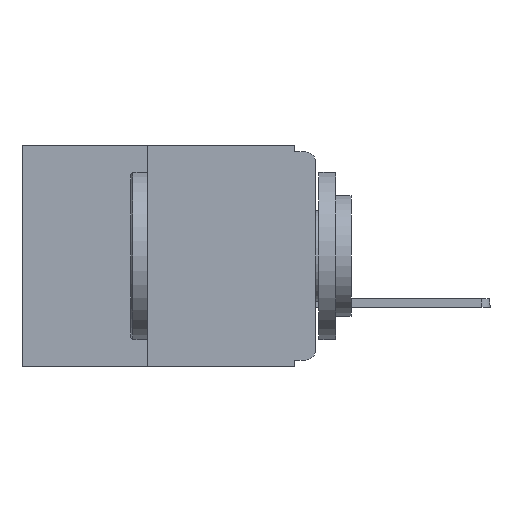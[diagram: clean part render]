
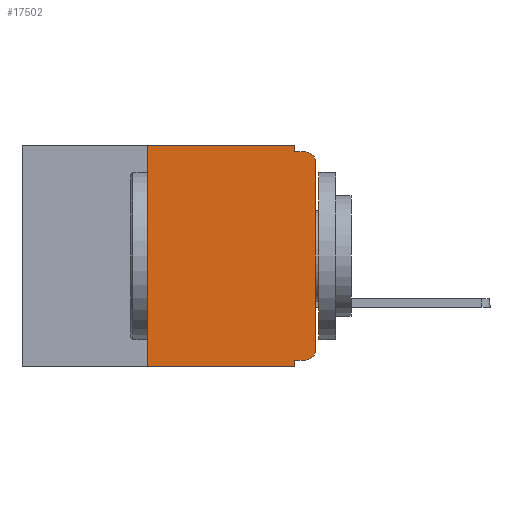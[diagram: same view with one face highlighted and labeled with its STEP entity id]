
A CAD part, left-side view. The second image highlights one B-rep face of the part: STEP entity #17502.
In plain terms, the highlighted planar face has unit normal (-1, 0, 0).
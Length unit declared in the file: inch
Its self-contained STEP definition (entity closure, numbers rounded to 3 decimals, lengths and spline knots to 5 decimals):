
#1093 = ORIENTED_EDGE ( 'NONE', *, *, #18024, .T. ) ;
#1341 = ORIENTED_EDGE ( 'NONE', *, *, #11001, .F. ) ;
#1710 = CARTESIAN_POINT ( 'NONE',  ( 0., 0.015, -0.025 ) ) ;
#1848 = CARTESIAN_POINT ( 'NONE',  ( 0., 0.015, -0.01 ) ) ;
#1984 = VERTEX_POINT ( 'NONE', #11458 ) ;
#2075 = CARTESIAN_POINT ( 'NONE',  ( 0., 0.031, 0. ) ) ;
#2078 = VERTEX_POINT ( 'NONE', #12396 ) ;
#2118 = ORIENTED_EDGE ( 'NONE', *, *, #21403, .F. ) ;
#3249 = ORIENTED_EDGE ( 'NONE', *, *, #15613, .F. ) ;
#3299 = LINE ( 'NONE', #16524, #12833 ) ;
#3483 = AXIS2_PLACEMENT_3D ( 'NONE', #1710, #14924, #3572 ) ;
#3572 = DIRECTION ( 'NONE',  ( 0., 0., -1. ) ) ;
#3679 = VERTEX_POINT ( 'NONE', #23639 ) ;
#3843 = VECTOR ( 'NONE', #21231, 39.37008 ) ;
#4228 = ORIENTED_EDGE ( 'NONE', *, *, #22177, .T. ) ;
#4853 = CARTESIAN_POINT ( 'NONE',  ( 0., 0., 0. ) ) ;
#5460 = DIRECTION ( 'NONE',  ( 0., 0., -1. ) ) ;
#5711 = AXIS2_PLACEMENT_3D ( 'NONE', #20771, #22678, #11487 ) ;
#6062 = CARTESIAN_POINT ( 'NONE',  ( 0., 0., -0.01 ) ) ;
#6402 = EDGE_LOOP ( 'NONE', ( #4228, #1093, #1341, #2118, #3249, #6449, #6737, #7347, #7793, #21954 ) ) ;
#6422 = EDGE_CURVE ( 'NONE', #16972, #3679, #21775, .T. ) ;
#6449 = ORIENTED_EDGE ( 'NONE', *, *, #18558, .F. ) ;
#6737 = ORIENTED_EDGE ( 'NONE', *, *, #16997, .T. ) ;
#7347 = ORIENTED_EDGE ( 'NONE', *, *, #11310, .F. ) ;
#7634 = PLANE ( 'NONE',  #5711 ) ;
#7793 = ORIENTED_EDGE ( 'NONE', *, *, #11449, .F. ) ;
#7931 = VECTOR ( 'NONE', #17489, 39.37008 ) ;
#8108 = CARTESIAN_POINT ( 'NONE',  ( 0., 0.437, 0. ) ) ;
#9319 = VERTEX_POINT ( 'NONE', #21881 ) ;
#9547 = LINE ( 'NONE', #6062, #3843 ) ;
#9656 = DIRECTION ( 'NONE',  ( 0., 1., 0. ) ) ;
#9844 = CARTESIAN_POINT ( 'NONE',  ( 0., 0., -0.025 ) ) ;
#10036 = DIRECTION ( 'NONE',  ( 0., -1., 0. ) ) ;
#10295 = VECTOR ( 'NONE', #18039, 39.37008 ) ;
#10493 = LINE ( 'NONE', #20041, #24250 ) ;
#10742 = DIRECTION ( 'NONE',  ( 0., -1., 0. ) ) ;
#10802 = VERTEX_POINT ( 'NONE', #1848 ) ;
#11001 = EDGE_CURVE ( 'NONE', #1984, #10802, #9547, .T. ) ;
#11310 = EDGE_CURVE ( 'NONE', #2078, #23770, #21860, .T. ) ;
#11338 = CIRCLE ( 'NONE', #3483, 0.015 ) ;
#11449 = EDGE_CURVE ( 'NONE', #16972, #2078, #14525, .T. ) ;
#11458 = CARTESIAN_POINT ( 'NONE',  ( 0., 0.031, -0.01 ) ) ;
#11487 = DIRECTION ( 'NONE',  ( 0., 0., -1. ) ) ;
#11511 = CARTESIAN_POINT ( 'NONE',  ( 0., 0., -0.32 ) ) ;
#11917 = CARTESIAN_POINT ( 'NONE',  ( 0., 0.031, 0. ) ) ;
#12396 = CARTESIAN_POINT ( 'NONE',  ( 0., 0.031, -0.32 ) ) ;
#12606 = LINE ( 'NONE', #8108, #16910 ) ;
#12833 = VECTOR ( 'NONE', #24019, 39.37008 ) ;
#12975 = LINE ( 'NONE', #11917, #7931 ) ;
#13433 = CARTESIAN_POINT ( 'NONE',  ( 0., 0.25, 0. ) ) ;
#13948 = VECTOR ( 'NONE', #9656, 39.37008 ) ;
#14525 = LINE ( 'NONE', #11511, #13948 ) ;
#14906 = VERTEX_POINT ( 'NONE', #13433 ) ;
#14924 = DIRECTION ( 'NONE',  ( -1., 0., 0. ) ) ;
#15613 = EDGE_CURVE ( 'NONE', #14906, #20009, #12606, .T. ) ;
#16524 = CARTESIAN_POINT ( 'NONE',  ( 0., 0.25, -0.33 ) ) ;
#16823 = VECTOR ( 'NONE', #5460, 39.37008 ) ;
#16910 = VECTOR ( 'NONE', #10036, 39.37008 ) ;
#16972 = VERTEX_POINT ( 'NONE', #23754 ) ;
#16997 = EDGE_CURVE ( 'NONE', #9319, #23770, #10493, .T. ) ;
#17489 = DIRECTION ( 'NONE',  ( 0., 0., -1. ) ) ;
#17502 = ADVANCED_FACE ( 'NONE', ( #18622 ), #7634, .F. ) ;
#18024 = EDGE_CURVE ( 'NONE', #22989, #10802, #11338, .T. ) ;
#18039 = DIRECTION ( 'NONE',  ( 0., 0., 1. ) ) ;
#18558 = EDGE_CURVE ( 'NONE', #9319, #14906, #3299, .T. ) ;
#18622 = FACE_OUTER_BOUND ( 'NONE', #6402, .T. ) ;
#19655 = LINE ( 'NONE', #4853, #10295 ) ;
#20009 = VERTEX_POINT ( 'NONE', #2075 ) ;
#20041 = CARTESIAN_POINT ( 'NONE',  ( 0., 0.437, -0.33 ) ) ;
#20771 = CARTESIAN_POINT ( 'NONE',  ( 0., 0.437, 0. ) ) ;
#21231 = DIRECTION ( 'NONE',  ( 0., -1., 0. ) ) ;
#21403 = EDGE_CURVE ( 'NONE', #20009, #1984, #12975, .T. ) ;
#21699 = CARTESIAN_POINT ( 'NONE',  ( 0., 0.031, -0.33 ) ) ;
#21775 = CIRCLE ( 'NONE', #24154, 0.015 ) ;
#21860 = LINE ( 'NONE', #24244, #16823 ) ;
#21881 = CARTESIAN_POINT ( 'NONE',  ( 0., 0.25, -0.33 ) ) ;
#21954 = ORIENTED_EDGE ( 'NONE', *, *, #6422, .T. ) ;
#22094 = DIRECTION ( 'NONE',  ( 0., 0., -1. ) ) ;
#22123 = CARTESIAN_POINT ( 'NONE',  ( 0., 0.015, -0.305 ) ) ;
#22167 = DIRECTION ( 'NONE',  ( -1., 0., 0. ) ) ;
#22177 = EDGE_CURVE ( 'NONE', #3679, #22989, #19655, .T. ) ;
#22678 = DIRECTION ( 'NONE',  ( 1., 0., 0. ) ) ;
#22989 = VERTEX_POINT ( 'NONE', #9844 ) ;
#23639 = CARTESIAN_POINT ( 'NONE',  ( 0., 0., -0.305 ) ) ;
#23754 = CARTESIAN_POINT ( 'NONE',  ( 0., 0.015, -0.32 ) ) ;
#23770 = VERTEX_POINT ( 'NONE', #21699 ) ;
#24019 = DIRECTION ( 'NONE',  ( 0., 0., 1. ) ) ;
#24154 = AXIS2_PLACEMENT_3D ( 'NONE', #22123, #22167, #22094 ) ;
#24244 = CARTESIAN_POINT ( 'NONE',  ( 0., 0.031, -0.33 ) ) ;
#24250 = VECTOR ( 'NONE', #10742, 39.37008 ) ;
